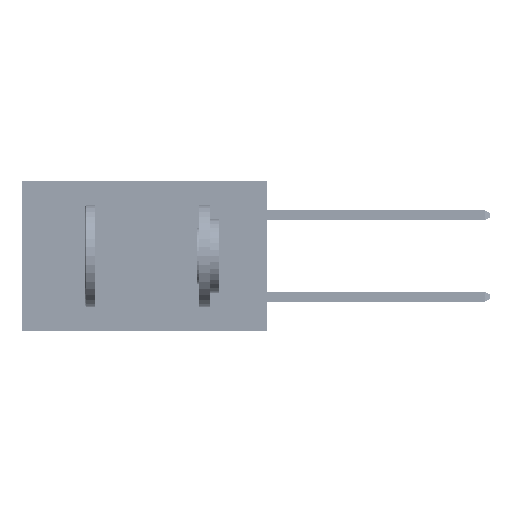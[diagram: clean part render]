
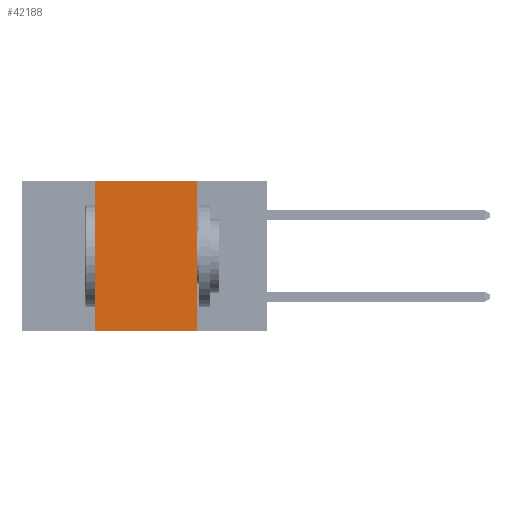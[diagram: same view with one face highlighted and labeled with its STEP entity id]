
A CAD part, left-side view. The second image highlights one B-rep face of the part: STEP entity #42188.
In plain terms, the highlighted planar face has unit normal (-1, 0, 0).
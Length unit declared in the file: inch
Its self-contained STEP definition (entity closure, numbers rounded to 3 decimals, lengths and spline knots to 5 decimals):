
#748 = EDGE_CURVE ( 'NONE', #21476, #40641, #20432, .T. ) ;
#2624 = EDGE_CURVE ( 'NONE', #21476, #42732, #7889, .T. ) ;
#3217 = AXIS2_PLACEMENT_3D ( 'NONE', #29561, #18474, #3729 ) ;
#3729 = DIRECTION ( 'NONE',  ( 0., 0., -1. ) ) ;
#5143 = CARTESIAN_POINT ( 'NONE',  ( 0., 0.6, -0.37 ) ) ;
#6980 = PLANE ( 'NONE',  #3217 ) ;
#7889 = LINE ( 'NONE', #19545, #42091 ) ;
#8420 = DIRECTION ( 'NONE',  ( 0., -1., 0. ) ) ;
#9724 = VERTEX_POINT ( 'NONE', #18004 ) ;
#11293 = LINE ( 'NONE', #18052, #33704 ) ;
#15848 = ORIENTED_EDGE ( 'NONE', *, *, #2624, .F. ) ;
#15897 = LINE ( 'NONE', #38560, #40648 ) ;
#17235 = ORIENTED_EDGE ( 'NONE', *, *, #28328, .F. ) ;
#18004 = CARTESIAN_POINT ( 'NONE',  ( 0., 0.17, 0. ) ) ;
#18052 = CARTESIAN_POINT ( 'NONE',  ( 0., 0.17, 0. ) ) ;
#18474 = DIRECTION ( 'NONE',  ( 1., 0., 0. ) ) ;
#19545 = CARTESIAN_POINT ( 'NONE',  ( 0., 0.42, 0. ) ) ;
#20432 = LINE ( 'NONE', #5143, #43452 ) ;
#21476 = VERTEX_POINT ( 'NONE', #35687 ) ;
#23798 = EDGE_LOOP ( 'NONE', ( #17235, #43780, #15848, #43874 ) ) ;
#28328 = EDGE_CURVE ( 'NONE', #9724, #40641, #11293, .T. ) ;
#29561 = CARTESIAN_POINT ( 'NONE',  ( 0., 0.6, 0. ) ) ;
#30698 = FACE_OUTER_BOUND ( 'NONE', #23798, .T. ) ;
#33704 = VECTOR ( 'NONE', #37364, 39.37008 ) ;
#35687 = CARTESIAN_POINT ( 'NONE',  ( 0., 0.42, -0.37 ) ) ;
#37364 = DIRECTION ( 'NONE',  ( 0., 0., -1. ) ) ;
#38560 = CARTESIAN_POINT ( 'NONE',  ( 0., 0.6, 0. ) ) ;
#40641 = VERTEX_POINT ( 'NONE', #42309 ) ;
#40648 = VECTOR ( 'NONE', #8420, 39.37008 ) ;
#42091 = VECTOR ( 'NONE', #42316, 39.37008 ) ;
#42174 = CARTESIAN_POINT ( 'NONE',  ( 0., 0.42, 0. ) ) ;
#42188 = ADVANCED_FACE ( 'NONE', ( #30698 ), #6980, .F. ) ;
#42309 = CARTESIAN_POINT ( 'NONE',  ( 0., 0.17, -0.37 ) ) ;
#42316 = DIRECTION ( 'NONE',  ( 0., 0., 1. ) ) ;
#42732 = VERTEX_POINT ( 'NONE', #42174 ) ;
#42764 = EDGE_CURVE ( 'NONE', #42732, #9724, #15897, .T. ) ;
#43452 = VECTOR ( 'NONE', #46963, 39.37008 ) ;
#43780 = ORIENTED_EDGE ( 'NONE', *, *, #42764, .F. ) ;
#43874 = ORIENTED_EDGE ( 'NONE', *, *, #748, .T. ) ;
#46963 = DIRECTION ( 'NONE',  ( 0., -1., 0. ) ) ;
